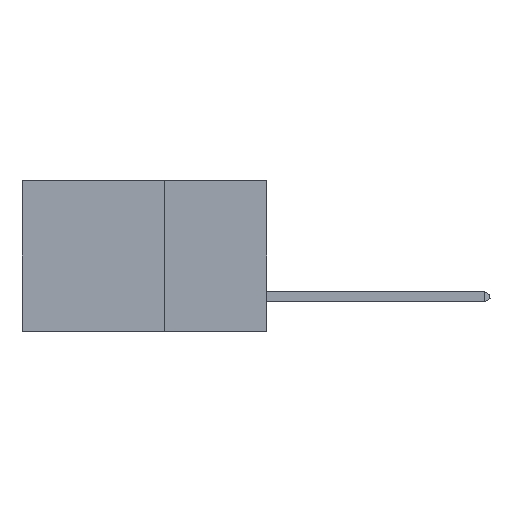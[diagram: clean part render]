
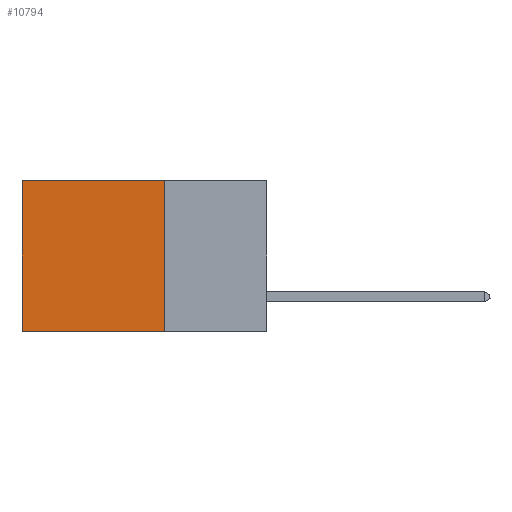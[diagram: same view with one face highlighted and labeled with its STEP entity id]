
A CAD part, left-side view. The second image highlights one B-rep face of the part: STEP entity #10794.
In plain terms, the highlighted planar face has unit normal (-1, 0, 0).
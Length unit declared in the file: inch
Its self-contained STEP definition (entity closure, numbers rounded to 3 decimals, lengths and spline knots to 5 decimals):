
#220 = CARTESIAN_POINT ( 'NONE',  ( 0.2875, 0.25, 0. ) ) ;
#359 = DIRECTION ( 'NONE',  ( 0., 0., -1. ) ) ;
#642 = EDGE_CURVE ( 'NONE', #5218, #23855, #21713, .T. ) ;
#1361 = CARTESIAN_POINT ( 'NONE',  ( 0.2875, 0.25, -0.37 ) ) ;
#1480 = CARTESIAN_POINT ( 'NONE',  ( 0.2875, 0.6, 0. ) ) ;
#5004 = LINE ( 'NONE', #7651, #9154 ) ;
#5134 = DIRECTION ( 'NONE',  ( 0., 1., 0. ) ) ;
#5218 = VERTEX_POINT ( 'NONE', #1480 ) ;
#5400 = ORIENTED_EDGE ( 'NONE', *, *, #20074, .T. ) ;
#5716 = EDGE_CURVE ( 'NONE', #27776, #23855, #9530, .T. ) ;
#7141 = VECTOR ( 'NONE', #22916, 39.37008 ) ;
#7300 = CARTESIAN_POINT ( 'NONE',  ( 0.2875, 0.6, -0.37 ) ) ;
#7651 = CARTESIAN_POINT ( 'NONE',  ( 0.2875, 0.25, 0. ) ) ;
#9154 = VECTOR ( 'NONE', #5134, 39.37008 ) ;
#9160 = VECTOR ( 'NONE', #25622, 39.37008 ) ;
#9323 = CARTESIAN_POINT ( 'NONE',  ( 0.2875, 0.25, 0. ) ) ;
#9530 = LINE ( 'NONE', #1361, #9160 ) ;
#10794 = ADVANCED_FACE ( 'NONE', ( #24641 ), #15678, .F. ) ;
#11377 = DIRECTION ( 'NONE',  ( 1., 0., 0. ) ) ;
#12632 = LINE ( 'NONE', #220, #16390 ) ;
#13366 = ORIENTED_EDGE ( 'NONE', *, *, #5716, .F. ) ;
#13633 = DIRECTION ( 'NONE',  ( 0., 0., -1. ) ) ;
#15678 = PLANE ( 'NONE',  #15883 ) ;
#15883 = AXIS2_PLACEMENT_3D ( 'NONE', #9323, #11377, #13633 ) ;
#15946 = CARTESIAN_POINT ( 'NONE',  ( 0.2875, 0.25, 0. ) ) ;
#16390 = VECTOR ( 'NONE', #359, 39.37008 ) ;
#17217 = VERTEX_POINT ( 'NONE', #15946 ) ;
#20074 = EDGE_CURVE ( 'NONE', #17217, #5218, #5004, .T. ) ;
#21291 = ORIENTED_EDGE ( 'NONE', *, *, #642, .T. ) ;
#21713 = LINE ( 'NONE', #26855, #7141 ) ;
#22916 = DIRECTION ( 'NONE',  ( 0., 0., -1. ) ) ;
#23085 = EDGE_CURVE ( 'NONE', #17217, #27776, #12632, .T. ) ;
#23855 = VERTEX_POINT ( 'NONE', #7300 ) ;
#24641 = FACE_OUTER_BOUND ( 'NONE', #26560, .T. ) ;
#25622 = DIRECTION ( 'NONE',  ( 0., 1., 0. ) ) ;
#26292 = ORIENTED_EDGE ( 'NONE', *, *, #23085, .F. ) ;
#26560 = EDGE_LOOP ( 'NONE', ( #21291, #13366, #26292, #5400 ) ) ;
#26855 = CARTESIAN_POINT ( 'NONE',  ( 0.2875, 0.6, 0. ) ) ;
#27122 = CARTESIAN_POINT ( 'NONE',  ( 0.2875, 0.25, -0.37 ) ) ;
#27776 = VERTEX_POINT ( 'NONE', #27122 ) ;
